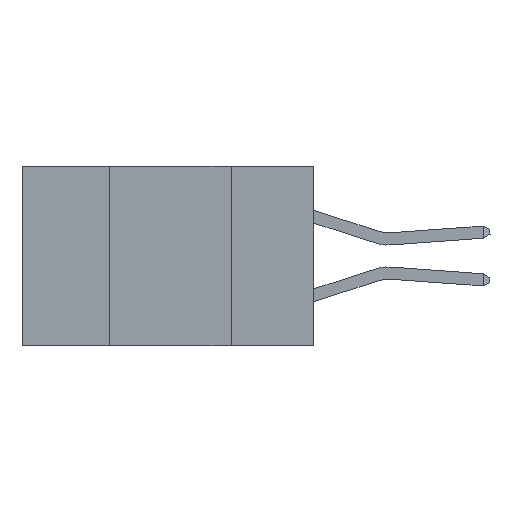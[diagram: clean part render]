
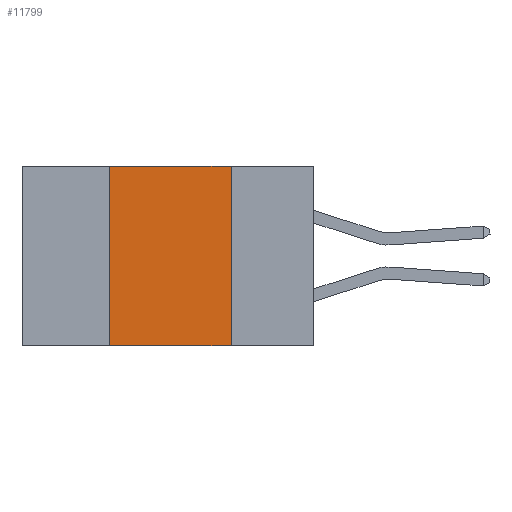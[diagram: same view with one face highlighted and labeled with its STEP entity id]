
A CAD part, left-side view. The second image highlights one B-rep face of the part: STEP entity #11799.
In plain terms, the highlighted planar face has unit normal (-1, 0, 0).
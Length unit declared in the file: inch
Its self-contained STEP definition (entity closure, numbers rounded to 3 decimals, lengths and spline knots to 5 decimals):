
#81 = PLANE ( 'NONE',  #1617 ) ;
#728 = LINE ( 'NONE', #4918, #8016 ) ;
#981 = CARTESIAN_POINT ( 'NONE',  ( 0., 0.17, 0. ) ) ;
#1617 = AXIS2_PLACEMENT_3D ( 'NONE', #7197, #15488, #5736 ) ;
#2136 = CARTESIAN_POINT ( 'NONE',  ( 0., 0.42, -0.37 ) ) ;
#2604 = ORIENTED_EDGE ( 'NONE', *, *, #7272, .F. ) ;
#2652 = FACE_OUTER_BOUND ( 'NONE', #17215, .T. ) ;
#3772 = LINE ( 'NONE', #9347, #10494 ) ;
#3960 = ORIENTED_EDGE ( 'NONE', *, *, #9365, .F. ) ;
#4220 = LINE ( 'NONE', #17967, #8233 ) ;
#4918 = CARTESIAN_POINT ( 'NONE',  ( 0., 0.17, 0. ) ) ;
#5736 = DIRECTION ( 'NONE',  ( 0., 0., -1. ) ) ;
#6962 = ORIENTED_EDGE ( 'NONE', *, *, #17339, .F. ) ;
#6985 = VECTOR ( 'NONE', #14442, 39.37008 ) ;
#7197 = CARTESIAN_POINT ( 'NONE',  ( 0., 0.6, 0. ) ) ;
#7272 = EDGE_CURVE ( 'NONE', #16042, #9480, #4220, .T. ) ;
#7920 = DIRECTION ( 'NONE',  ( 0., 0., -1. ) ) ;
#8016 = VECTOR ( 'NONE', #7920, 39.37008 ) ;
#8233 = VECTOR ( 'NONE', #15236, 39.37008 ) ;
#9347 = CARTESIAN_POINT ( 'NONE',  ( 0., 0.6, -0.37 ) ) ;
#9365 = EDGE_CURVE ( 'NONE', #13892, #14555, #728, .T. ) ;
#9480 = VERTEX_POINT ( 'NONE', #17754 ) ;
#10255 = CARTESIAN_POINT ( 'NONE',  ( 0., 0.6, 0. ) ) ;
#10494 = VECTOR ( 'NONE', #10791, 39.37008 ) ;
#10791 = DIRECTION ( 'NONE',  ( 0., -1., 0. ) ) ;
#11799 = ADVANCED_FACE ( 'NONE', ( #2652 ), #81, .F. ) ;
#11884 = LINE ( 'NONE', #10255, #6985 ) ;
#13798 = CARTESIAN_POINT ( 'NONE',  ( 0., 0.17, -0.37 ) ) ;
#13892 = VERTEX_POINT ( 'NONE', #981 ) ;
#14442 = DIRECTION ( 'NONE',  ( 0., -1., 0. ) ) ;
#14555 = VERTEX_POINT ( 'NONE', #13798 ) ;
#15236 = DIRECTION ( 'NONE',  ( 0., 0., 1. ) ) ;
#15488 = DIRECTION ( 'NONE',  ( 1., 0., 0. ) ) ;
#15611 = ORIENTED_EDGE ( 'NONE', *, *, #17528, .T. ) ;
#16042 = VERTEX_POINT ( 'NONE', #2136 ) ;
#17215 = EDGE_LOOP ( 'NONE', ( #3960, #6962, #2604, #15611 ) ) ;
#17339 = EDGE_CURVE ( 'NONE', #9480, #13892, #11884, .T. ) ;
#17528 = EDGE_CURVE ( 'NONE', #16042, #14555, #3772, .T. ) ;
#17754 = CARTESIAN_POINT ( 'NONE',  ( 0., 0.42, 0. ) ) ;
#17967 = CARTESIAN_POINT ( 'NONE',  ( 0., 0.42, 0. ) ) ;
